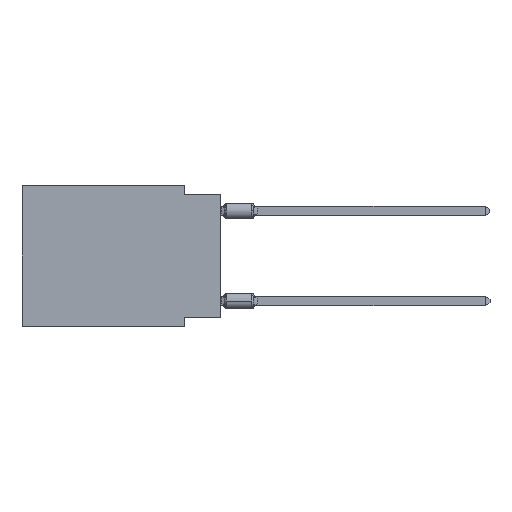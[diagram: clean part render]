
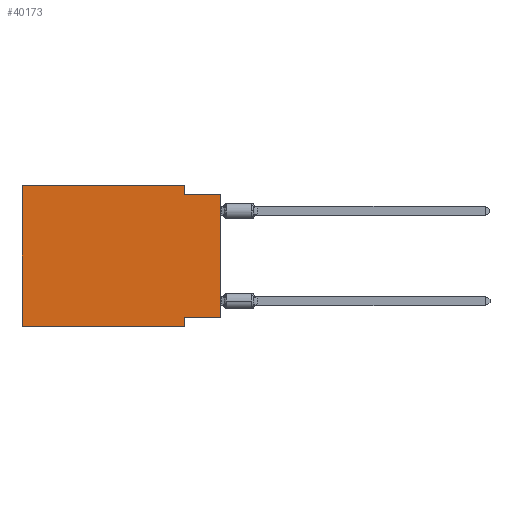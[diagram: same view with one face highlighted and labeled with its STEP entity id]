
A CAD part, left-side view. The second image highlights one B-rep face of the part: STEP entity #40173.
In plain terms, the highlighted planar face has unit normal (-1, 0, 0).
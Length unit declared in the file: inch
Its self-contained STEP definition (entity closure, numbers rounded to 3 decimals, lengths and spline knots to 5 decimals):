
#296 = ORIENTED_EDGE ( 'NONE', *, *, #12875, .F. ) ;
#555 = ORIENTED_EDGE ( 'NONE', *, *, #40472, .F. ) ;
#967 = VERTEX_POINT ( 'NONE', #8418 ) ;
#1557 = EDGE_CURVE ( 'NONE', #6880, #55305, #45152, .T. ) ;
#5163 = DIRECTION ( 'NONE',  ( 0., 0., -1. ) ) ;
#5441 = DIRECTION ( 'NONE',  ( 0., -1., 0. ) ) ;
#6122 = LINE ( 'NONE', #24409, #6711 ) ;
#6519 = CARTESIAN_POINT ( 'NONE',  ( 0., 0.1, -0.39 ) ) ;
#6711 = VECTOR ( 'NONE', #29206, 39.37008 ) ;
#6863 = CARTESIAN_POINT ( 'NONE',  ( 0., 0.55, 0. ) ) ;
#6880 = VERTEX_POINT ( 'NONE', #16594 ) ;
#7961 = VERTEX_POINT ( 'NONE', #6519 ) ;
#8418 = CARTESIAN_POINT ( 'NONE',  ( 0., 0.55, -0.39 ) ) ;
#9157 = LINE ( 'NONE', #36141, #51201 ) ;
#9476 = DIRECTION ( 'NONE',  ( 0., 0., -1. ) ) ;
#10336 = CARTESIAN_POINT ( 'NONE',  ( 0., 0.55, -0.39 ) ) ;
#10880 = CARTESIAN_POINT ( 'NONE',  ( 0., 0.1, -0.025 ) ) ;
#11922 = VECTOR ( 'NONE', #26109, 39.37008 ) ;
#12875 = EDGE_CURVE ( 'NONE', #967, #41103, #47945, .T. ) ;
#13450 = EDGE_CURVE ( 'NONE', #45574, #50390, #6122, .T. ) ;
#13951 = LINE ( 'NONE', #10336, #47092 ) ;
#15704 = EDGE_CURVE ( 'NONE', #967, #7961, #13951, .T. ) ;
#16527 = ORIENTED_EDGE ( 'NONE', *, *, #36437, .F. ) ;
#16594 = CARTESIAN_POINT ( 'NONE',  ( 0., 0.1, 0. ) ) ;
#18534 = ORIENTED_EDGE ( 'NONE', *, *, #22366, .F. ) ;
#22366 = EDGE_CURVE ( 'NONE', #41103, #6880, #23418, .T. ) ;
#23418 = LINE ( 'NONE', #27932, #56090 ) ;
#24409 = CARTESIAN_POINT ( 'NONE',  ( 0., 0., 0. ) ) ;
#25824 = LINE ( 'NONE', #43793, #11922 ) ;
#26109 = DIRECTION ( 'NONE',  ( 0., 1., 0. ) ) ;
#26844 = ORIENTED_EDGE ( 'NONE', *, *, #29087, .F. ) ;
#27932 = CARTESIAN_POINT ( 'NONE',  ( 0., 0.55, 0. ) ) ;
#29087 = EDGE_CURVE ( 'NONE', #55305, #50390, #35222, .T. ) ;
#29206 = DIRECTION ( 'NONE',  ( 0., 0., 1. ) ) ;
#31559 = FACE_OUTER_BOUND ( 'NONE', #42653, .T. ) ;
#32446 = DIRECTION ( 'NONE',  ( 1., 0., 0. ) ) ;
#33734 = CARTESIAN_POINT ( 'NONE',  ( 0., 0., -0.025 ) ) ;
#34623 = DIRECTION ( 'NONE',  ( 0., -1., 0. ) ) ;
#35222 = LINE ( 'NONE', #48738, #57421 ) ;
#35258 = ORIENTED_EDGE ( 'NONE', *, *, #13450, .T. ) ;
#36141 = CARTESIAN_POINT ( 'NONE',  ( 0., 0.1, -0.39 ) ) ;
#36437 = EDGE_CURVE ( 'NONE', #45186, #7961, #9157, .T. ) ;
#40173 = ADVANCED_FACE ( 'NONE', ( #31559 ), #41150, .F. ) ;
#40472 = EDGE_CURVE ( 'NONE', #45574, #45186, #25824, .T. ) ;
#40904 = CARTESIAN_POINT ( 'NONE',  ( 0., 0., -0.365 ) ) ;
#40940 = DIRECTION ( 'NONE',  ( 0., 0., -1. ) ) ;
#41103 = VERTEX_POINT ( 'NONE', #48411 ) ;
#41150 = PLANE ( 'NONE',  #58003 ) ;
#42653 = EDGE_LOOP ( 'NONE', ( #35258, #26844, #51637, #18534, #296, #54519, #16527, #555 ) ) ;
#43793 = CARTESIAN_POINT ( 'NONE',  ( 0., 0., -0.365 ) ) ;
#44010 = DIRECTION ( 'NONE',  ( 0., 0., 1. ) ) ;
#45152 = LINE ( 'NONE', #55041, #49899 ) ;
#45186 = VERTEX_POINT ( 'NONE', #59227 ) ;
#45574 = VERTEX_POINT ( 'NONE', #40904 ) ;
#47092 = VECTOR ( 'NONE', #55028, 39.37008 ) ;
#47945 = LINE ( 'NONE', #6863, #58491 ) ;
#48411 = CARTESIAN_POINT ( 'NONE',  ( 0., 0.55, 0. ) ) ;
#48738 = CARTESIAN_POINT ( 'NONE',  ( 0., 0., -0.025 ) ) ;
#49899 = VECTOR ( 'NONE', #9476, 39.37008 ) ;
#50390 = VERTEX_POINT ( 'NONE', #33734 ) ;
#51201 = VECTOR ( 'NONE', #40940, 39.37008 ) ;
#51637 = ORIENTED_EDGE ( 'NONE', *, *, #1557, .F. ) ;
#54519 = ORIENTED_EDGE ( 'NONE', *, *, #15704, .T. ) ;
#55028 = DIRECTION ( 'NONE',  ( 0., -1., 0. ) ) ;
#55041 = CARTESIAN_POINT ( 'NONE',  ( 0., 0.1, 0. ) ) ;
#55238 = CARTESIAN_POINT ( 'NONE',  ( 0., 0.55, 0. ) ) ;
#55305 = VERTEX_POINT ( 'NONE', #10880 ) ;
#56090 = VECTOR ( 'NONE', #5441, 39.37008 ) ;
#57421 = VECTOR ( 'NONE', #34623, 39.37008 ) ;
#58003 = AXIS2_PLACEMENT_3D ( 'NONE', #55238, #32446, #5163 ) ;
#58491 = VECTOR ( 'NONE', #44010, 39.37008 ) ;
#59227 = CARTESIAN_POINT ( 'NONE',  ( 0., 0.1, -0.365 ) ) ;
